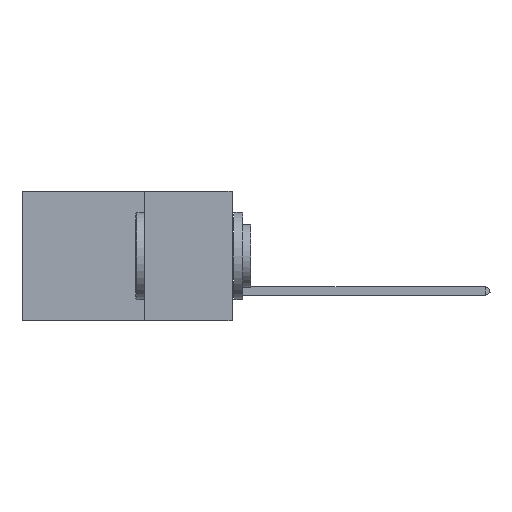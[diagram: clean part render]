
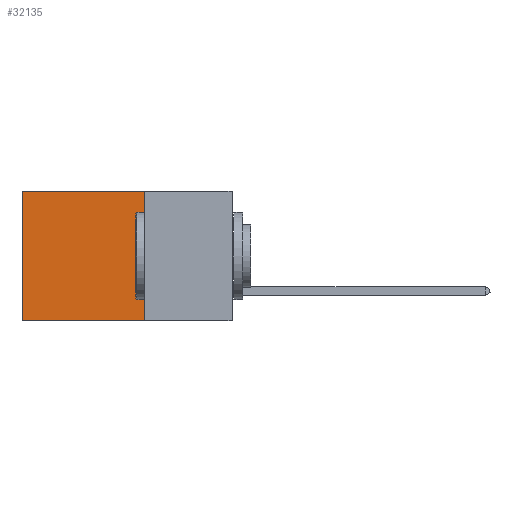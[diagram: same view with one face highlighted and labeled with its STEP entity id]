
A CAD part, left-side view. The second image highlights one B-rep face of the part: STEP entity #32135.
In plain terms, the highlighted planar face has unit normal (-1, 0, 0).
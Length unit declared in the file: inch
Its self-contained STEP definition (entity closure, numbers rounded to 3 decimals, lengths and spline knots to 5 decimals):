
#2946 = DIRECTION ( 'NONE',  ( 1., 0., 0. ) ) ;
#3939 = DIRECTION ( 'NONE',  ( 0., 0., -1. ) ) ;
#6578 = ORIENTED_EDGE ( 'NONE', *, *, #43626, .T. ) ;
#7109 = LINE ( 'NONE', #7158, #33686 ) ;
#7158 = CARTESIAN_POINT ( 'NONE',  ( 0.2875, 0.25, 0. ) ) ;
#11928 = EDGE_LOOP ( 'NONE', ( #14375, #21590, #34522, #6578 ) ) ;
#12175 = VERTEX_POINT ( 'NONE', #31870 ) ;
#12987 = CARTESIAN_POINT ( 'NONE',  ( 0.2875, 0.25, -0.37 ) ) ;
#14052 = VECTOR ( 'NONE', #3939, 39.37008 ) ;
#14349 = EDGE_CURVE ( 'NONE', #12175, #34433, #42011, .T. ) ;
#14375 = ORIENTED_EDGE ( 'NONE', *, *, #20730, .T. ) ;
#15065 = CARTESIAN_POINT ( 'NONE',  ( 0.2875, 0.25, 0. ) ) ;
#16191 = CARTESIAN_POINT ( 'NONE',  ( 0.2875, 0.6, 0. ) ) ;
#17312 = PLANE ( 'NONE',  #40088 ) ;
#19607 = DIRECTION ( 'NONE',  ( 0., 0., -1. ) ) ;
#20730 = EDGE_CURVE ( 'NONE', #46432, #34433, #36656, .T. ) ;
#21590 = ORIENTED_EDGE ( 'NONE', *, *, #14349, .F. ) ;
#22491 = FACE_OUTER_BOUND ( 'NONE', #11928, .T. ) ;
#25452 = CARTESIAN_POINT ( 'NONE',  ( 0.2875, 0.6, 0. ) ) ;
#26251 = CARTESIAN_POINT ( 'NONE',  ( 0.2875, 0.6, -0.37 ) ) ;
#27287 = VECTOR ( 'NONE', #42390, 39.37008 ) ;
#28395 = EDGE_CURVE ( 'NONE', #43252, #12175, #35008, .T. ) ;
#31870 = CARTESIAN_POINT ( 'NONE',  ( 0.2875, 0.25, -0.37 ) ) ;
#32015 = DIRECTION ( 'NONE',  ( 0., 0., -1. ) ) ;
#32135 = ADVANCED_FACE ( 'NONE', ( #22491 ), #17312, .F. ) ;
#32425 = DIRECTION ( 'NONE',  ( 0., 1., 0. ) ) ;
#33686 = VECTOR ( 'NONE', #32425, 39.37008 ) ;
#34433 = VERTEX_POINT ( 'NONE', #26251 ) ;
#34522 = ORIENTED_EDGE ( 'NONE', *, *, #28395, .F. ) ;
#35008 = LINE ( 'NONE', #36661, #14052 ) ;
#36656 = LINE ( 'NONE', #25452, #37246 ) ;
#36661 = CARTESIAN_POINT ( 'NONE',  ( 0.2875, 0.25, 0. ) ) ;
#37246 = VECTOR ( 'NONE', #19607, 39.37008 ) ;
#40088 = AXIS2_PLACEMENT_3D ( 'NONE', #46614, #2946, #32015 ) ;
#42011 = LINE ( 'NONE', #12987, #27287 ) ;
#42390 = DIRECTION ( 'NONE',  ( 0., 1., 0. ) ) ;
#43252 = VERTEX_POINT ( 'NONE', #15065 ) ;
#43626 = EDGE_CURVE ( 'NONE', #43252, #46432, #7109, .T. ) ;
#46432 = VERTEX_POINT ( 'NONE', #16191 ) ;
#46614 = CARTESIAN_POINT ( 'NONE',  ( 0.2875, 0.25, 0. ) ) ;
